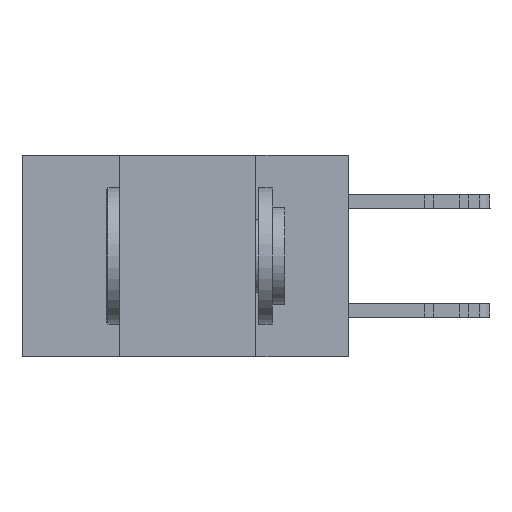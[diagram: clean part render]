
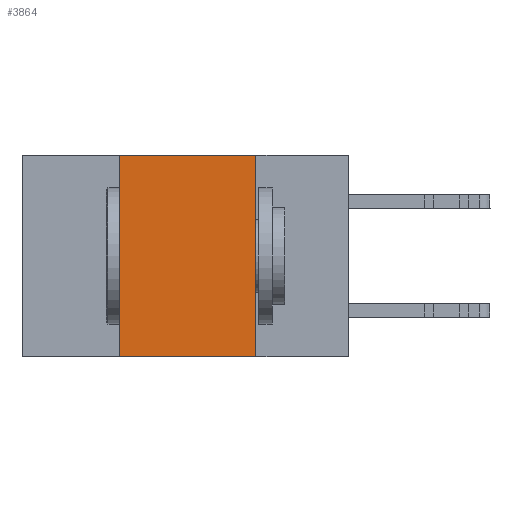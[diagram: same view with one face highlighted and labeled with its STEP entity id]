
A CAD part, left-side view. The second image highlights one B-rep face of the part: STEP entity #3864.
In plain terms, the highlighted planar face has unit normal (-1, 0, 0).
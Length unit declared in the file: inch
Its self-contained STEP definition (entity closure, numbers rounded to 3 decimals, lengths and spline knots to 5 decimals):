
#112 = DIRECTION ( 'NONE',  ( 0., -1., 0. ) ) ;
#1011 = CARTESIAN_POINT ( 'NONE',  ( 0., 0.6, -0.37 ) ) ;
#2737 = EDGE_CURVE ( 'NONE', #10806, #17627, #9078, .T. ) ;
#3515 = ORIENTED_EDGE ( 'NONE', *, *, #8196, .T. ) ;
#3701 = AXIS2_PLACEMENT_3D ( 'NONE', #17174, #17047, #19212 ) ;
#3864 = ADVANCED_FACE ( 'NONE', ( #22778 ), #9151, .F. ) ;
#4125 = VECTOR ( 'NONE', #22211, 39.37008 ) ;
#5584 = LINE ( 'NONE', #19023, #10231 ) ;
#5697 = DIRECTION ( 'NONE',  ( 0., 0., -1. ) ) ;
#5764 = ORIENTED_EDGE ( 'NONE', *, *, #17132, .F. ) ;
#7263 = ORIENTED_EDGE ( 'NONE', *, *, #2737, .F. ) ;
#8196 = EDGE_CURVE ( 'NONE', #24878, #14613, #13310, .T. ) ;
#8763 = EDGE_LOOP ( 'NONE', ( #5764, #7263, #16862, #3515 ) ) ;
#9078 = LINE ( 'NONE', #10498, #4125 ) ;
#9141 = DIRECTION ( 'NONE',  ( 0., 0., 1. ) ) ;
#9151 = PLANE ( 'NONE',  #3701 ) ;
#10231 = VECTOR ( 'NONE', #5697, 39.37008 ) ;
#10498 = CARTESIAN_POINT ( 'NONE',  ( 0., 0.6, 0. ) ) ;
#10694 = EDGE_CURVE ( 'NONE', #24878, #10806, #22766, .T. ) ;
#10806 = VERTEX_POINT ( 'NONE', #16921 ) ;
#11628 = VECTOR ( 'NONE', #112, 39.37008 ) ;
#13310 = LINE ( 'NONE', #1011, #11628 ) ;
#14613 = VERTEX_POINT ( 'NONE', #21312 ) ;
#15418 = CARTESIAN_POINT ( 'NONE',  ( 0., 0.42, -0.37 ) ) ;
#16862 = ORIENTED_EDGE ( 'NONE', *, *, #10694, .F. ) ;
#16921 = CARTESIAN_POINT ( 'NONE',  ( 0., 0.42, 0. ) ) ;
#17047 = DIRECTION ( 'NONE',  ( 1., 0., 0. ) ) ;
#17132 = EDGE_CURVE ( 'NONE', #17627, #14613, #5584, .T. ) ;
#17174 = CARTESIAN_POINT ( 'NONE',  ( 0., 0.6, 0. ) ) ;
#17627 = VERTEX_POINT ( 'NONE', #18732 ) ;
#18732 = CARTESIAN_POINT ( 'NONE',  ( 0., 0.17, 0. ) ) ;
#18971 = CARTESIAN_POINT ( 'NONE',  ( 0., 0.42, -0.37 ) ) ;
#19023 = CARTESIAN_POINT ( 'NONE',  ( 0., 0.17, -0.37 ) ) ;
#19212 = DIRECTION ( 'NONE',  ( 0., 0., -1. ) ) ;
#20651 = VECTOR ( 'NONE', #9141, 39.37008 ) ;
#21312 = CARTESIAN_POINT ( 'NONE',  ( 0., 0.17, -0.37 ) ) ;
#22211 = DIRECTION ( 'NONE',  ( 0., -1., 0. ) ) ;
#22766 = LINE ( 'NONE', #18971, #20651 ) ;
#22778 = FACE_OUTER_BOUND ( 'NONE', #8763, .T. ) ;
#24878 = VERTEX_POINT ( 'NONE', #15418 ) ;
